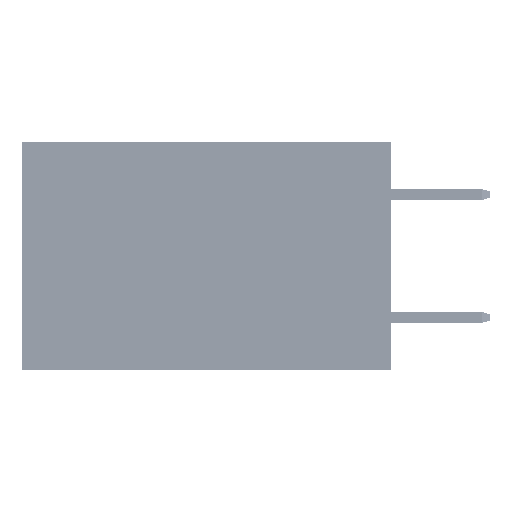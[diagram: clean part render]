
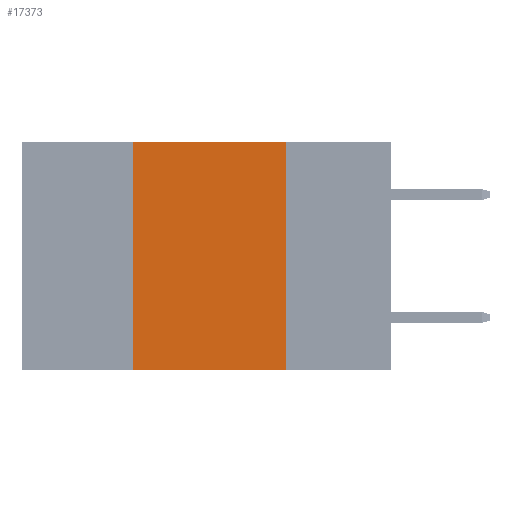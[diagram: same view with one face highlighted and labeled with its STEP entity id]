
A CAD part, left-side view. The second image highlights one B-rep face of the part: STEP entity #17373.
In plain terms, the highlighted planar face has unit normal (-1, 0, 0).
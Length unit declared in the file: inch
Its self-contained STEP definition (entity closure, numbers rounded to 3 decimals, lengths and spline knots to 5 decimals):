
#540 = VERTEX_POINT ( 'NONE', #6019 ) ;
#1349 = CARTESIAN_POINT ( 'NONE',  ( 0., 0.17, -0.37 ) ) ;
#1468 = CARTESIAN_POINT ( 'NONE',  ( 0., 0.17, 0. ) ) ;
#2291 = VECTOR ( 'NONE', #5061, 39.37008 ) ;
#3077 = CARTESIAN_POINT ( 'NONE',  ( 0., 0.42, -0.37 ) ) ;
#4014 = LINE ( 'NONE', #1468, #2291 ) ;
#4412 = FACE_OUTER_BOUND ( 'NONE', #40169, .T. ) ;
#4856 = VERTEX_POINT ( 'NONE', #1349 ) ;
#4937 = VERTEX_POINT ( 'NONE', #8127 ) ;
#5061 = DIRECTION ( 'NONE',  ( 0., 0., -1. ) ) ;
#5094 = CARTESIAN_POINT ( 'NONE',  ( 0., 0.42, 0. ) ) ;
#6019 = CARTESIAN_POINT ( 'NONE',  ( 0., 0.17, 0. ) ) ;
#6056 = DIRECTION ( 'NONE',  ( 1., 0., 0. ) ) ;
#6781 = ORIENTED_EDGE ( 'NONE', *, *, #36185, .F. ) ;
#7346 = LINE ( 'NONE', #5094, #16177 ) ;
#7814 = ORIENTED_EDGE ( 'NONE', *, *, #13021, .F. ) ;
#8127 = CARTESIAN_POINT ( 'NONE',  ( 0., 0.42, 0. ) ) ;
#8128 = CARTESIAN_POINT ( 'NONE',  ( 0., 0.6, -0.37 ) ) ;
#13021 = EDGE_CURVE ( 'NONE', #4937, #540, #46581, .T. ) ;
#15157 = ORIENTED_EDGE ( 'NONE', *, *, #40116, .F. ) ;
#16177 = VECTOR ( 'NONE', #46860, 39.37008 ) ;
#17373 = ADVANCED_FACE ( 'NONE', ( #4412 ), #43347, .F. ) ;
#18587 = CARTESIAN_POINT ( 'NONE',  ( 0., 0.6, 0. ) ) ;
#20364 = VERTEX_POINT ( 'NONE', #3077 ) ;
#20554 = VECTOR ( 'NONE', #42140, 39.37008 ) ;
#21175 = DIRECTION ( 'NONE',  ( 0., 0., -1. ) ) ;
#23603 = VECTOR ( 'NONE', #44867, 39.37008 ) ;
#30336 = ORIENTED_EDGE ( 'NONE', *, *, #43525, .T. ) ;
#30855 = AXIS2_PLACEMENT_3D ( 'NONE', #32208, #6056, #21175 ) ;
#32208 = CARTESIAN_POINT ( 'NONE',  ( 0., 0.6, 0. ) ) ;
#36185 = EDGE_CURVE ( 'NONE', #540, #4856, #4014, .T. ) ;
#40116 = EDGE_CURVE ( 'NONE', #20364, #4937, #7346, .T. ) ;
#40169 = EDGE_LOOP ( 'NONE', ( #6781, #7814, #15157, #30336 ) ) ;
#42140 = DIRECTION ( 'NONE',  ( 0., -1., 0. ) ) ;
#43347 = PLANE ( 'NONE',  #30855 ) ;
#43525 = EDGE_CURVE ( 'NONE', #20364, #4856, #45827, .T. ) ;
#44867 = DIRECTION ( 'NONE',  ( 0., -1., 0. ) ) ;
#45827 = LINE ( 'NONE', #8128, #20554 ) ;
#46581 = LINE ( 'NONE', #18587, #23603 ) ;
#46860 = DIRECTION ( 'NONE',  ( 0., 0., 1. ) ) ;
